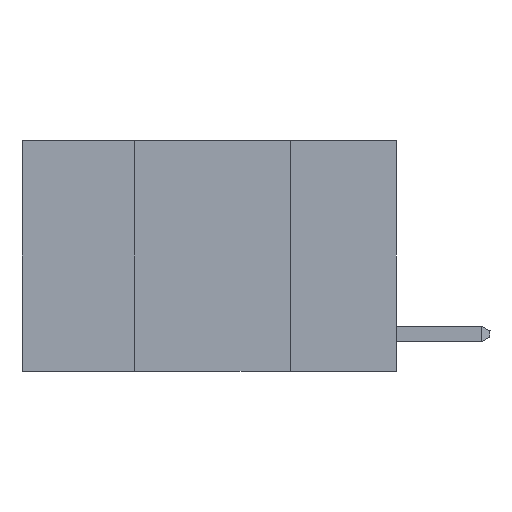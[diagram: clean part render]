
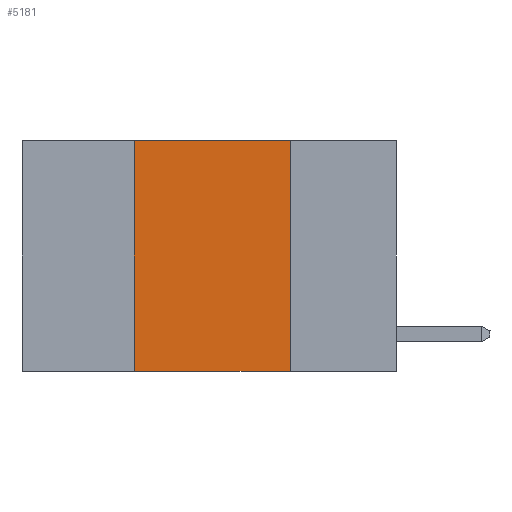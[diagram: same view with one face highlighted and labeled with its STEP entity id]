
A CAD part, left-side view. The second image highlights one B-rep face of the part: STEP entity #5181.
In plain terms, the highlighted planar face has unit normal (-1, 0, 0).
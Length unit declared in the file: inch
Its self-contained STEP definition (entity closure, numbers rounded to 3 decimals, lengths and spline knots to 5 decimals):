
#1204 = EDGE_CURVE ( 'NONE', #4313, #5173, #11992, .T. ) ;
#1225 = CARTESIAN_POINT ( 'NONE',  ( 0., 0.42, -0.37 ) ) ;
#1445 = FACE_OUTER_BOUND ( 'NONE', #5543, .T. ) ;
#1761 = DIRECTION ( 'NONE',  ( 0., -1., 0. ) ) ;
#2268 = CARTESIAN_POINT ( 'NONE',  ( 0., 0.17, 0. ) ) ;
#3389 = CARTESIAN_POINT ( 'NONE',  ( 0., 0.6, 0. ) ) ;
#4313 = VERTEX_POINT ( 'NONE', #2268 ) ;
#4422 = ORIENTED_EDGE ( 'NONE', *, *, #6193, .F. ) ;
#4664 = EDGE_CURVE ( 'NONE', #5656, #5173, #11668, .T. ) ;
#4873 = ORIENTED_EDGE ( 'NONE', *, *, #1204, .F. ) ;
#5173 = VERTEX_POINT ( 'NONE', #6459 ) ;
#5181 = ADVANCED_FACE ( 'NONE', ( #1445 ), #6253, .F. ) ;
#5543 = EDGE_LOOP ( 'NONE', ( #4873, #4422, #13910, #8422 ) ) ;
#5656 = VERTEX_POINT ( 'NONE', #1225 ) ;
#6193 = EDGE_CURVE ( 'NONE', #9727, #4313, #13370, .T. ) ;
#6253 = PLANE ( 'NONE',  #10473 ) ;
#6459 = CARTESIAN_POINT ( 'NONE',  ( 0., 0.17, -0.37 ) ) ;
#7142 = DIRECTION ( 'NONE',  ( 0., 0., 1. ) ) ;
#7156 = EDGE_CURVE ( 'NONE', #5656, #9727, #14397, .T. ) ;
#7278 = DIRECTION ( 'NONE',  ( 0., 0., -1. ) ) ;
#7410 = CARTESIAN_POINT ( 'NONE',  ( 0., 0.6, -0.37 ) ) ;
#7420 = DIRECTION ( 'NONE',  ( 0., 0., -1. ) ) ;
#8101 = VECTOR ( 'NONE', #11389, 39.37008 ) ;
#8422 = ORIENTED_EDGE ( 'NONE', *, *, #4664, .T. ) ;
#9287 = CARTESIAN_POINT ( 'NONE',  ( 0., 0.42, 0. ) ) ;
#9557 = VECTOR ( 'NONE', #1761, 39.37008 ) ;
#9727 = VERTEX_POINT ( 'NONE', #10872 ) ;
#10473 = AXIS2_PLACEMENT_3D ( 'NONE', #12057, #14171, #7420 ) ;
#10872 = CARTESIAN_POINT ( 'NONE',  ( 0., 0.42, 0. ) ) ;
#11389 = DIRECTION ( 'NONE',  ( 0., -1., 0. ) ) ;
#11668 = LINE ( 'NONE', #7410, #9557 ) ;
#11992 = LINE ( 'NONE', #13924, #14101 ) ;
#12057 = CARTESIAN_POINT ( 'NONE',  ( 0., 0.6, 0. ) ) ;
#12827 = VECTOR ( 'NONE', #7142, 39.37008 ) ;
#13370 = LINE ( 'NONE', #3389, #8101 ) ;
#13910 = ORIENTED_EDGE ( 'NONE', *, *, #7156, .F. ) ;
#13924 = CARTESIAN_POINT ( 'NONE',  ( 0., 0.17, 0. ) ) ;
#14101 = VECTOR ( 'NONE', #7278, 39.37008 ) ;
#14171 = DIRECTION ( 'NONE',  ( 1., 0., 0. ) ) ;
#14397 = LINE ( 'NONE', #9287, #12827 ) ;
